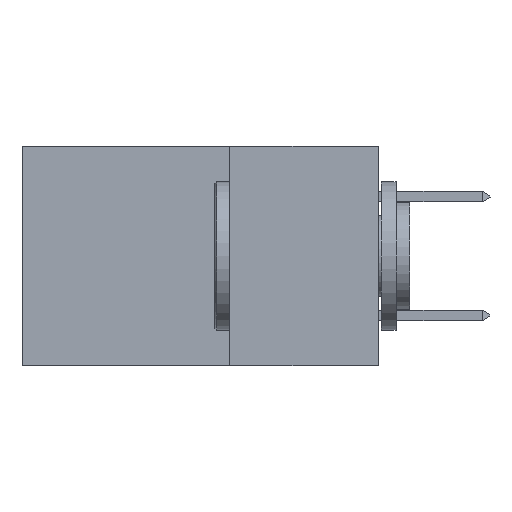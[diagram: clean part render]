
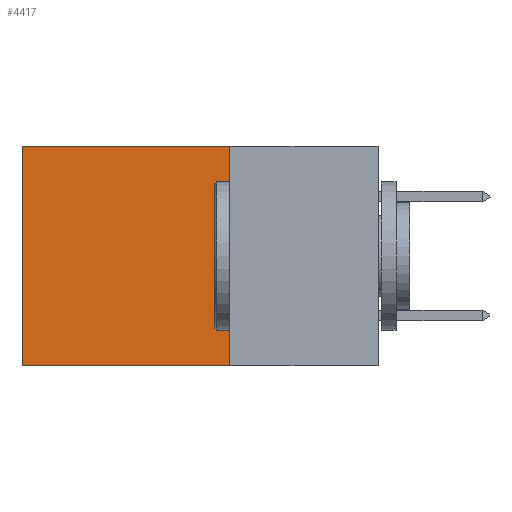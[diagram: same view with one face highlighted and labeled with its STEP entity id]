
A CAD part, left-side view. The second image highlights one B-rep face of the part: STEP entity #4417.
In plain terms, the highlighted planar face has unit normal (-1, 0, 0).
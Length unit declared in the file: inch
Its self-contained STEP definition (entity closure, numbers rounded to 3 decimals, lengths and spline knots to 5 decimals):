
#200 = VECTOR ( 'NONE', #20618, 39.37008 ) ;
#235 = CARTESIAN_POINT ( 'NONE',  ( 0.298, 0.25, -0.37 ) ) ;
#394 = PLANE ( 'NONE',  #8683 ) ;
#1494 = VECTOR ( 'NONE', #7648, 39.37008 ) ;
#3583 = VERTEX_POINT ( 'NONE', #11939 ) ;
#3704 = VERTEX_POINT ( 'NONE', #9955 ) ;
#3802 = DIRECTION ( 'NONE',  ( 1., 0., 0. ) ) ;
#4148 = ORIENTED_EDGE ( 'NONE', *, *, #17783, .F. ) ;
#4417 = ADVANCED_FACE ( 'NONE', ( #8055 ), #394, .F. ) ;
#5538 = DIRECTION ( 'NONE',  ( 0., 1., 0. ) ) ;
#7648 = DIRECTION ( 'NONE',  ( 0., 0., -1. ) ) ;
#8055 = FACE_OUTER_BOUND ( 'NONE', #10189, .T. ) ;
#8683 = AXIS2_PLACEMENT_3D ( 'NONE', #18909, #3802, #15544 ) ;
#8878 = EDGE_CURVE ( 'NONE', #12385, #3704, #18035, .T. ) ;
#9310 = VECTOR ( 'NONE', #5538, 39.37008 ) ;
#9831 = LINE ( 'NONE', #13703, #9310 ) ;
#9955 = CARTESIAN_POINT ( 'NONE',  ( 0.298, 0.6, -0.37 ) ) ;
#10105 = DIRECTION ( 'NONE',  ( 0., 0., -1. ) ) ;
#10189 = EDGE_LOOP ( 'NONE', ( #17015, #4148, #20872, #18153 ) ) ;
#10560 = EDGE_CURVE ( 'NONE', #3583, #12385, #9831, .T. ) ;
#11242 = EDGE_CURVE ( 'NONE', #3583, #16481, #11389, .T. ) ;
#11389 = LINE ( 'NONE', #14885, #12984 ) ;
#11939 = CARTESIAN_POINT ( 'NONE',  ( 0.298, 0.25, 0. ) ) ;
#11974 = CARTESIAN_POINT ( 'NONE',  ( 0.298, 0.25, -0.37 ) ) ;
#12042 = LINE ( 'NONE', #11974, #200 ) ;
#12385 = VERTEX_POINT ( 'NONE', #14355 ) ;
#12984 = VECTOR ( 'NONE', #10105, 39.37008 ) ;
#13703 = CARTESIAN_POINT ( 'NONE',  ( 0.298, 0.25, 0. ) ) ;
#14355 = CARTESIAN_POINT ( 'NONE',  ( 0.298, 0.6, 0. ) ) ;
#14885 = CARTESIAN_POINT ( 'NONE',  ( 0.298, 0.25, 0. ) ) ;
#15544 = DIRECTION ( 'NONE',  ( 0., 0., -1. ) ) ;
#16481 = VERTEX_POINT ( 'NONE', #235 ) ;
#17015 = ORIENTED_EDGE ( 'NONE', *, *, #8878, .T. ) ;
#17783 = EDGE_CURVE ( 'NONE', #16481, #3704, #12042, .T. ) ;
#18035 = LINE ( 'NONE', #20966, #1494 ) ;
#18153 = ORIENTED_EDGE ( 'NONE', *, *, #10560, .T. ) ;
#18909 = CARTESIAN_POINT ( 'NONE',  ( 0.298, 0.25, 0. ) ) ;
#20618 = DIRECTION ( 'NONE',  ( 0., 1., 0. ) ) ;
#20872 = ORIENTED_EDGE ( 'NONE', *, *, #11242, .F. ) ;
#20966 = CARTESIAN_POINT ( 'NONE',  ( 0.298, 0.6, 0. ) ) ;
